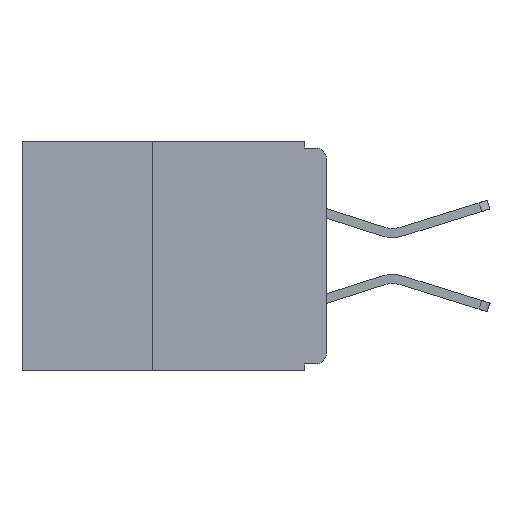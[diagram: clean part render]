
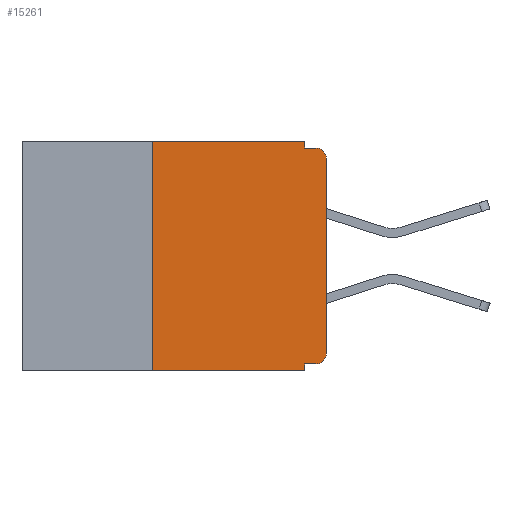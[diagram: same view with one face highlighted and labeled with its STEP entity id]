
A CAD part, left-side view. The second image highlights one B-rep face of the part: STEP entity #15261.
In plain terms, the highlighted planar face has unit normal (-1, 0, 0).
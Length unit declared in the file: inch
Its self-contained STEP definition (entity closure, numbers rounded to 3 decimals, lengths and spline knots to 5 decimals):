
#858 = AXIS2_PLACEMENT_3D ( 'NONE', #27632, #12400, #30094 ) ;
#1670 = VECTOR ( 'NONE', #16414, 39.37008 ) ;
#1680 = VERTEX_POINT ( 'NONE', #29140 ) ;
#1912 = LINE ( 'NONE', #13760, #26879 ) ;
#2752 = DIRECTION ( 'NONE',  ( -1., 0., 0. ) ) ;
#2980 = EDGE_CURVE ( 'NONE', #5844, #32383, #1912, .T. ) ;
#3401 = ORIENTED_EDGE ( 'NONE', *, *, #31742, .T. ) ;
#3496 = PLANE ( 'NONE',  #17358 ) ;
#3783 = CARTESIAN_POINT ( 'NONE',  ( 0., 0., -0.025 ) ) ;
#3912 = CARTESIAN_POINT ( 'NONE',  ( 0., 0.437, 0. ) ) ;
#3949 = VERTEX_POINT ( 'NONE', #10179 ) ;
#5241 = DIRECTION ( 'NONE',  ( 0., 0., -1. ) ) ;
#5375 = CARTESIAN_POINT ( 'NONE',  ( 0., 0., -0.305 ) ) ;
#5390 = VECTOR ( 'NONE', #26263, 39.37008 ) ;
#5844 = VERTEX_POINT ( 'NONE', #20616 ) ;
#6567 = CIRCLE ( 'NONE', #13875, 0.015 ) ;
#6653 = EDGE_LOOP ( 'NONE', ( #12005, #21635, #12436, #8130, #29593, #15071, #15537, #25302, #12207, #3401 ) ) ;
#6877 = FACE_OUTER_BOUND ( 'NONE', #6653, .T. ) ;
#8130 = ORIENTED_EDGE ( 'NONE', *, *, #32068, .F. ) ;
#8193 = VECTOR ( 'NONE', #27152, 39.37008 ) ;
#8328 = LINE ( 'NONE', #20050, #21230 ) ;
#9479 = LINE ( 'NONE', #26478, #1670 ) ;
#10179 = CARTESIAN_POINT ( 'NONE',  ( 0., 0.031, -0.32 ) ) ;
#10263 = CARTESIAN_POINT ( 'NONE',  ( 0., 0.031, 0. ) ) ;
#10602 = CARTESIAN_POINT ( 'NONE',  ( 0., 0., 0. ) ) ;
#11075 = LINE ( 'NONE', #3912, #18011 ) ;
#11391 = CARTESIAN_POINT ( 'NONE',  ( 0., 0.015, -0.32 ) ) ;
#11491 = EDGE_CURVE ( 'NONE', #11945, #3949, #8328, .T. ) ;
#11785 = EDGE_CURVE ( 'NONE', #16457, #1680, #19264, .T. ) ;
#11945 = VERTEX_POINT ( 'NONE', #11391 ) ;
#12005 = ORIENTED_EDGE ( 'NONE', *, *, #24814, .T. ) ;
#12207 = ORIENTED_EDGE ( 'NONE', *, *, #11491, .F. ) ;
#12400 = DIRECTION ( 'NONE',  ( -1., 0., 0. ) ) ;
#12436 = ORIENTED_EDGE ( 'NONE', *, *, #2980, .F. ) ;
#12467 = EDGE_CURVE ( 'NONE', #3949, #32873, #21177, .T. ) ;
#13232 = DIRECTION ( 'NONE',  ( 0., 0., 1. ) ) ;
#13579 = CARTESIAN_POINT ( 'NONE',  ( 0., 0.25, -0.33 ) ) ;
#13760 = CARTESIAN_POINT ( 'NONE',  ( 0., 0., -0.01 ) ) ;
#13875 = AXIS2_PLACEMENT_3D ( 'NONE', #18369, #2752, #20930 ) ;
#14110 = CARTESIAN_POINT ( 'NONE',  ( 0., 0.437, 0. ) ) ;
#14223 = DIRECTION ( 'NONE',  ( 0., 0., -1. ) ) ;
#14238 = DIRECTION ( 'NONE',  ( 0., -1., 0. ) ) ;
#15071 = ORIENTED_EDGE ( 'NONE', *, *, #11785, .F. ) ;
#15261 = ADVANCED_FACE ( 'NONE', ( #6877 ), #3496, .F. ) ;
#15537 = ORIENTED_EDGE ( 'NONE', *, *, #21088, .T. ) ;
#15644 = CARTESIAN_POINT ( 'NONE',  ( 0., 0.031, -0.33 ) ) ;
#16414 = DIRECTION ( 'NONE',  ( 0., -1., 0. ) ) ;
#16457 = VERTEX_POINT ( 'NONE', #28865 ) ;
#16926 = DIRECTION ( 'NONE',  ( 0., -1., 0. ) ) ;
#17005 = CARTESIAN_POINT ( 'NONE',  ( 0., 0.031, 0. ) ) ;
#17358 = AXIS2_PLACEMENT_3D ( 'NONE', #14110, #29356, #14223 ) ;
#17850 = VERTEX_POINT ( 'NONE', #3783 ) ;
#18011 = VECTOR ( 'NONE', #16926, 39.37008 ) ;
#18369 = CARTESIAN_POINT ( 'NONE',  ( 0., 0.015, -0.305 ) ) ;
#19264 = LINE ( 'NONE', #13579, #5390 ) ;
#19468 = VERTEX_POINT ( 'NONE', #10263 ) ;
#20050 = CARTESIAN_POINT ( 'NONE',  ( 0., 0., -0.32 ) ) ;
#20616 = CARTESIAN_POINT ( 'NONE',  ( 0., 0.031, -0.01 ) ) ;
#20930 = DIRECTION ( 'NONE',  ( 0., 0., -1. ) ) ;
#21088 = EDGE_CURVE ( 'NONE', #16457, #32873, #9479, .T. ) ;
#21177 = LINE ( 'NONE', #15644, #27050 ) ;
#21230 = VECTOR ( 'NONE', #22558, 39.37008 ) ;
#21635 = ORIENTED_EDGE ( 'NONE', *, *, #27528, .T. ) ;
#22558 = DIRECTION ( 'NONE',  ( 0., 1., 0. ) ) ;
#23818 = EDGE_CURVE ( 'NONE', #1680, #19468, #11075, .T. ) ;
#24814 = EDGE_CURVE ( 'NONE', #31761, #17850, #28598, .T. ) ;
#25302 = ORIENTED_EDGE ( 'NONE', *, *, #12467, .F. ) ;
#26263 = DIRECTION ( 'NONE',  ( 0., 0., 1. ) ) ;
#26478 = CARTESIAN_POINT ( 'NONE',  ( 0., 0.437, -0.33 ) ) ;
#26657 = CARTESIAN_POINT ( 'NONE',  ( 0., 0.015, -0.01 ) ) ;
#26734 = CARTESIAN_POINT ( 'NONE',  ( 0., 0.031, -0.33 ) ) ;
#26879 = VECTOR ( 'NONE', #14238, 39.37008 ) ;
#27050 = VECTOR ( 'NONE', #5241, 39.37008 ) ;
#27152 = DIRECTION ( 'NONE',  ( 0., 0., -1. ) ) ;
#27528 = EDGE_CURVE ( 'NONE', #17850, #32383, #31050, .T. ) ;
#27632 = CARTESIAN_POINT ( 'NONE',  ( 0., 0.015, -0.025 ) ) ;
#27839 = VECTOR ( 'NONE', #13232, 39.37008 ) ;
#28598 = LINE ( 'NONE', #10602, #27839 ) ;
#28865 = CARTESIAN_POINT ( 'NONE',  ( 0., 0.25, -0.33 ) ) ;
#29140 = CARTESIAN_POINT ( 'NONE',  ( 0., 0.25, 0. ) ) ;
#29299 = LINE ( 'NONE', #17005, #8193 ) ;
#29356 = DIRECTION ( 'NONE',  ( 1., 0., 0. ) ) ;
#29593 = ORIENTED_EDGE ( 'NONE', *, *, #23818, .F. ) ;
#30094 = DIRECTION ( 'NONE',  ( 0., 0., -1. ) ) ;
#31050 = CIRCLE ( 'NONE', #858, 0.015 ) ;
#31742 = EDGE_CURVE ( 'NONE', #11945, #31761, #6567, .T. ) ;
#31761 = VERTEX_POINT ( 'NONE', #5375 ) ;
#32068 = EDGE_CURVE ( 'NONE', #19468, #5844, #29299, .T. ) ;
#32383 = VERTEX_POINT ( 'NONE', #26657 ) ;
#32873 = VERTEX_POINT ( 'NONE', #26734 ) ;
